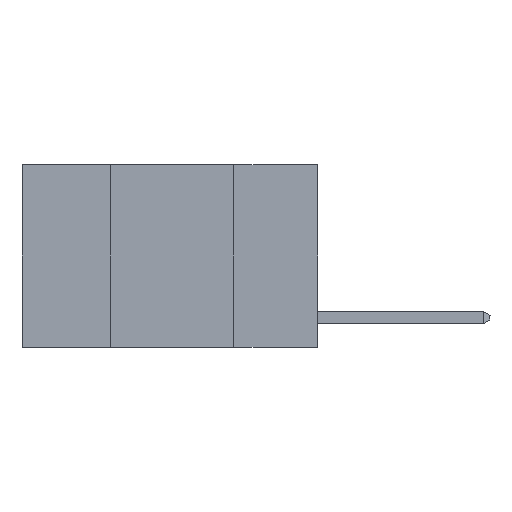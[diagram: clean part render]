
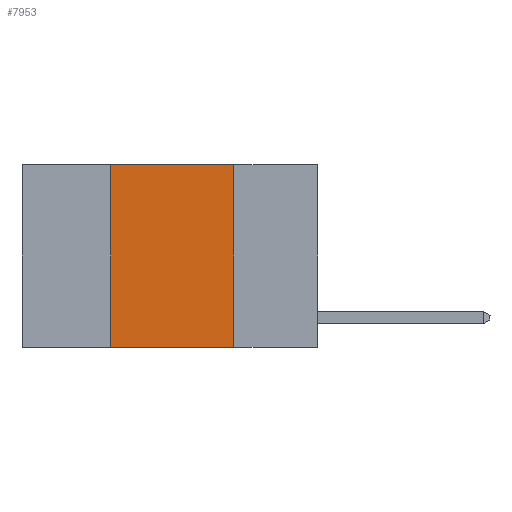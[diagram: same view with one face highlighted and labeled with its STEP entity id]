
A CAD part, left-side view. The second image highlights one B-rep face of the part: STEP entity #7953.
In plain terms, the highlighted planar face has unit normal (-1, 0, 0).
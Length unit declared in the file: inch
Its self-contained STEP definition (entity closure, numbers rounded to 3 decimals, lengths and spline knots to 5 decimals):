
#116 = VERTEX_POINT ( 'NONE', #14794 ) ;
#1239 = ORIENTED_EDGE ( 'NONE', *, *, #14485, .F. ) ;
#2288 = FACE_OUTER_BOUND ( 'NONE', #8731, .T. ) ;
#2543 = ORIENTED_EDGE ( 'NONE', *, *, #23119, .F. ) ;
#3492 = EDGE_CURVE ( 'NONE', #20547, #16660, #8274, .T. ) ;
#5369 = CARTESIAN_POINT ( 'NONE',  ( 0., 0.6, 0. ) ) ;
#6963 = AXIS2_PLACEMENT_3D ( 'NONE', #5369, #20957, #7623 ) ;
#7623 = DIRECTION ( 'NONE',  ( 0., 0., -1. ) ) ;
#7953 = ADVANCED_FACE ( 'NONE', ( #2288 ), #18701, .F. ) ;
#8274 = LINE ( 'NONE', #17544, #14162 ) ;
#8731 = EDGE_LOOP ( 'NONE', ( #2543, #1239, #18352, #9599 ) ) ;
#8952 = VERTEX_POINT ( 'NONE', #11530 ) ;
#9043 = CARTESIAN_POINT ( 'NONE',  ( 0., 0.17, 0. ) ) ;
#9599 = ORIENTED_EDGE ( 'NONE', *, *, #26458, .T. ) ;
#10265 = CARTESIAN_POINT ( 'NONE',  ( 0., 0.6, -0.37 ) ) ;
#11262 = DIRECTION ( 'NONE',  ( 0., 0., -1. ) ) ;
#11530 = CARTESIAN_POINT ( 'NONE',  ( 0., 0.17, 0. ) ) ;
#12935 = VECTOR ( 'NONE', #25850, 39.37008 ) ;
#14162 = VECTOR ( 'NONE', #22004, 39.37008 ) ;
#14485 = EDGE_CURVE ( 'NONE', #16660, #8952, #21295, .T. ) ;
#14794 = CARTESIAN_POINT ( 'NONE',  ( 0., 0.17, -0.37 ) ) ;
#16660 = VERTEX_POINT ( 'NONE', #28325 ) ;
#17544 = CARTESIAN_POINT ( 'NONE',  ( 0., 0.42, 0. ) ) ;
#18170 = LINE ( 'NONE', #10265, #12935 ) ;
#18229 = DIRECTION ( 'NONE',  ( 0., -1., 0. ) ) ;
#18352 = ORIENTED_EDGE ( 'NONE', *, *, #3492, .F. ) ;
#18701 = PLANE ( 'NONE',  #6963 ) ;
#20547 = VERTEX_POINT ( 'NONE', #24425 ) ;
#20957 = DIRECTION ( 'NONE',  ( 1., 0., 0. ) ) ;
#21139 = LINE ( 'NONE', #9043, #27061 ) ;
#21295 = LINE ( 'NONE', #22719, #26526 ) ;
#22004 = DIRECTION ( 'NONE',  ( 0., 0., 1. ) ) ;
#22719 = CARTESIAN_POINT ( 'NONE',  ( 0., 0.6, 0. ) ) ;
#23119 = EDGE_CURVE ( 'NONE', #8952, #116, #21139, .T. ) ;
#24425 = CARTESIAN_POINT ( 'NONE',  ( 0., 0.42, -0.37 ) ) ;
#25850 = DIRECTION ( 'NONE',  ( 0., -1., 0. ) ) ;
#26458 = EDGE_CURVE ( 'NONE', #20547, #116, #18170, .T. ) ;
#26526 = VECTOR ( 'NONE', #18229, 39.37008 ) ;
#27061 = VECTOR ( 'NONE', #11262, 39.37008 ) ;
#28325 = CARTESIAN_POINT ( 'NONE',  ( 0., 0.42, 0. ) ) ;
